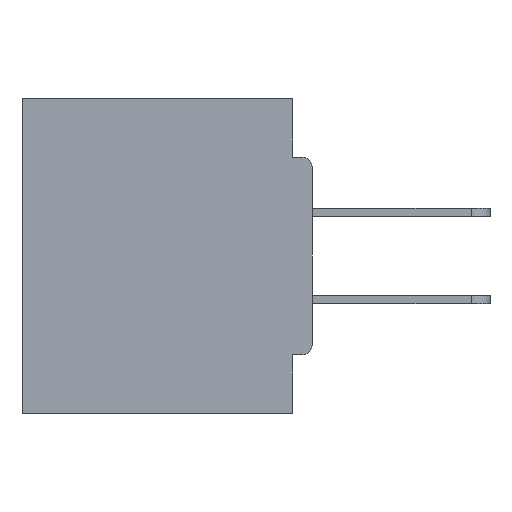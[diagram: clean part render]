
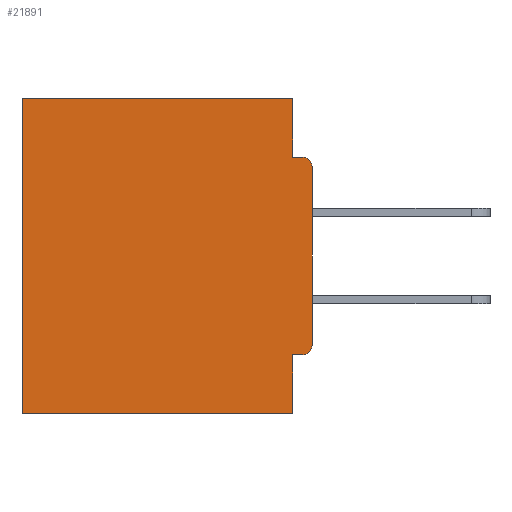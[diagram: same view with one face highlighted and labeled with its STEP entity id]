
A CAD part, left-side view. The second image highlights one B-rep face of the part: STEP entity #21891.
In plain terms, the highlighted planar face has unit normal (-1, 0, 0).
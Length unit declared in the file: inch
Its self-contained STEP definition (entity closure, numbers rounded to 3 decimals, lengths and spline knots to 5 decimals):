
#1446 = VERTEX_POINT ( 'NONE', #30755 ) ;
#1984 = CIRCLE ( 'NONE', #13661, 0.015 ) ;
#2457 = CARTESIAN_POINT ( 'NONE',  ( 0.298, 0.46, 0. ) ) ;
#2465 = DIRECTION ( 'NONE',  ( 0., 0., -1. ) ) ;
#2936 = CARTESIAN_POINT ( 'NONE',  ( 0.298, 0., -0.0935 ) ) ;
#3595 = CARTESIAN_POINT ( 'NONE',  ( 0.298, 0., 0. ) ) ;
#3624 = ORIENTED_EDGE ( 'NONE', *, *, #26590, .T. ) ;
#3672 = VECTOR ( 'NONE', #23249, 39.37008 ) ;
#3898 = LINE ( 'NONE', #10206, #20914 ) ;
#4096 = EDGE_CURVE ( 'NONE', #25597, #23624, #3898, .T. ) ;
#4348 = FACE_OUTER_BOUND ( 'NONE', #30169, .T. ) ;
#4506 = DIRECTION ( 'NONE',  ( 0., 0., -1. ) ) ;
#4519 = DIRECTION ( 'NONE',  ( 0., 1., 0. ) ) ;
#4725 = VECTOR ( 'NONE', #25828, 39.37008 ) ;
#4920 = EDGE_CURVE ( 'NONE', #25597, #28057, #21277, .T. ) ;
#5039 = PLANE ( 'NONE',  #31443 ) ;
#6160 = LINE ( 'NONE', #29968, #14086 ) ;
#6367 = ORIENTED_EDGE ( 'NONE', *, *, #10509, .F. ) ;
#7056 = AXIS2_PLACEMENT_3D ( 'NONE', #9570, #12239, #19550 ) ;
#7709 = LINE ( 'NONE', #3595, #11717 ) ;
#8243 = LINE ( 'NONE', #2936, #4725 ) ;
#8551 = ORIENTED_EDGE ( 'NONE', *, *, #11826, .T. ) ;
#8821 = EDGE_CURVE ( 'NONE', #23624, #8866, #6160, .T. ) ;
#8866 = VERTEX_POINT ( 'NONE', #26460 ) ;
#9567 = VERTEX_POINT ( 'NONE', #10899 ) ;
#9570 = CARTESIAN_POINT ( 'NONE',  ( 0.298, 0.015, -0.1085 ) ) ;
#10206 = CARTESIAN_POINT ( 'NONE',  ( 0.298, 0., 0. ) ) ;
#10361 = LINE ( 'NONE', #25554, #3672 ) ;
#10509 = EDGE_CURVE ( 'NONE', #24665, #1446, #30015, .T. ) ;
#10676 = DIRECTION ( 'NONE',  ( 0., 0., -1. ) ) ;
#10899 = CARTESIAN_POINT ( 'NONE',  ( 0.298, 0.015, -0.0935 ) ) ;
#11058 = CARTESIAN_POINT ( 'NONE',  ( 0.298, 0., -0.1085 ) ) ;
#11660 = VECTOR ( 'NONE', #4519, 39.37008 ) ;
#11717 = VECTOR ( 'NONE', #21091, 39.37008 ) ;
#11826 = EDGE_CURVE ( 'NONE', #20693, #9567, #24472, .T. ) ;
#12206 = VECTOR ( 'NONE', #10676, 39.37008 ) ;
#12239 = DIRECTION ( 'NONE',  ( -1., 0., 0. ) ) ;
#12671 = DIRECTION ( 'NONE',  ( 0., 1., 0. ) ) ;
#12802 = DIRECTION ( 'NONE',  ( 1., 0., 0. ) ) ;
#13099 = ORIENTED_EDGE ( 'NONE', *, *, #18694, .F. ) ;
#13661 = AXIS2_PLACEMENT_3D ( 'NONE', #19382, #14089, #14207 ) ;
#14086 = VECTOR ( 'NONE', #2465, 39.37008 ) ;
#14089 = DIRECTION ( 'NONE',  ( -1., 0., 0. ) ) ;
#14207 = DIRECTION ( 'NONE',  ( 0., 0., -1. ) ) ;
#14535 = VECTOR ( 'NONE', #4506, 39.37008 ) ;
#16171 = CARTESIAN_POINT ( 'NONE',  ( 0.298, 0.031, 0. ) ) ;
#17986 = VERTEX_POINT ( 'NONE', #26159 ) ;
#17990 = EDGE_CURVE ( 'NONE', #20693, #17986, #7709, .T. ) ;
#18694 = EDGE_CURVE ( 'NONE', #22310, #24665, #29483, .T. ) ;
#19382 = CARTESIAN_POINT ( 'NONE',  ( 0.298, 0.015, -0.3915 ) ) ;
#19550 = DIRECTION ( 'NONE',  ( 0., 0., -1. ) ) ;
#19866 = CARTESIAN_POINT ( 'NONE',  ( 0.298, 0., -0.4065 ) ) ;
#20693 = VERTEX_POINT ( 'NONE', #11058 ) ;
#20914 = VECTOR ( 'NONE', #12671, 39.37008 ) ;
#21091 = DIRECTION ( 'NONE',  ( 0., 0., -1. ) ) ;
#21277 = LINE ( 'NONE', #30073, #14535 ) ;
#21804 = ORIENTED_EDGE ( 'NONE', *, *, #31117, .F. ) ;
#21891 = ADVANCED_FACE ( 'NONE', ( #4348 ), #5039, .F. ) ;
#22310 = VERTEX_POINT ( 'NONE', #27152 ) ;
#23249 = DIRECTION ( 'NONE',  ( 0., 1., 0. ) ) ;
#23624 = VERTEX_POINT ( 'NONE', #2457 ) ;
#23727 = EDGE_CURVE ( 'NONE', #1446, #8866, #10361, .T. ) ;
#23856 = ORIENTED_EDGE ( 'NONE', *, *, #4096, .T. ) ;
#24472 = CIRCLE ( 'NONE', #7056, 0.015 ) ;
#24665 = VERTEX_POINT ( 'NONE', #30160 ) ;
#25398 = CARTESIAN_POINT ( 'NONE',  ( 0.298, 0., 0. ) ) ;
#25512 = DIRECTION ( 'NONE',  ( 0., 0., -1. ) ) ;
#25554 = CARTESIAN_POINT ( 'NONE',  ( 0.298, 0., -0.5 ) ) ;
#25597 = VERTEX_POINT ( 'NONE', #16171 ) ;
#25828 = DIRECTION ( 'NONE',  ( 0., -1., 0. ) ) ;
#25874 = CARTESIAN_POINT ( 'NONE',  ( 0.298, 0.031, -0.5 ) ) ;
#26159 = CARTESIAN_POINT ( 'NONE',  ( 0.298, 0., -0.3915 ) ) ;
#26460 = CARTESIAN_POINT ( 'NONE',  ( 0.298, 0.46, -0.5 ) ) ;
#26590 = EDGE_CURVE ( 'NONE', #22310, #17986, #1984, .T. ) ;
#26737 = ORIENTED_EDGE ( 'NONE', *, *, #4920, .F. ) ;
#27152 = CARTESIAN_POINT ( 'NONE',  ( 0.298, 0.015, -0.4065 ) ) ;
#27493 = CARTESIAN_POINT ( 'NONE',  ( 0.298, 0.031, -0.0935 ) ) ;
#27856 = ORIENTED_EDGE ( 'NONE', *, *, #23727, .F. ) ;
#27899 = ORIENTED_EDGE ( 'NONE', *, *, #17990, .F. ) ;
#28057 = VERTEX_POINT ( 'NONE', #27493 ) ;
#29483 = LINE ( 'NONE', #19866, #11660 ) ;
#29968 = CARTESIAN_POINT ( 'NONE',  ( 0.298, 0.46, 0. ) ) ;
#30015 = LINE ( 'NONE', #25874, #12206 ) ;
#30073 = CARTESIAN_POINT ( 'NONE',  ( 0.298, 0.031, -0.5 ) ) ;
#30160 = CARTESIAN_POINT ( 'NONE',  ( 0.298, 0.031, -0.4065 ) ) ;
#30169 = EDGE_LOOP ( 'NONE', ( #8551, #21804, #26737, #23856, #31869, #27856, #6367, #13099, #3624, #27899 ) ) ;
#30755 = CARTESIAN_POINT ( 'NONE',  ( 0.298, 0.031, -0.5 ) ) ;
#31117 = EDGE_CURVE ( 'NONE', #28057, #9567, #8243, .T. ) ;
#31443 = AXIS2_PLACEMENT_3D ( 'NONE', #25398, #12802, #25512 ) ;
#31869 = ORIENTED_EDGE ( 'NONE', *, *, #8821, .T. ) ;
